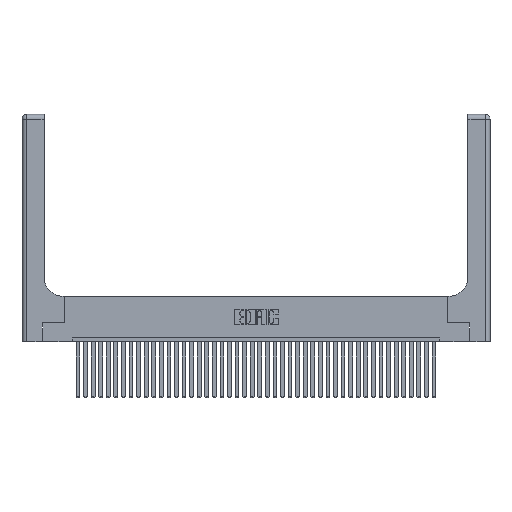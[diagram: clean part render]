
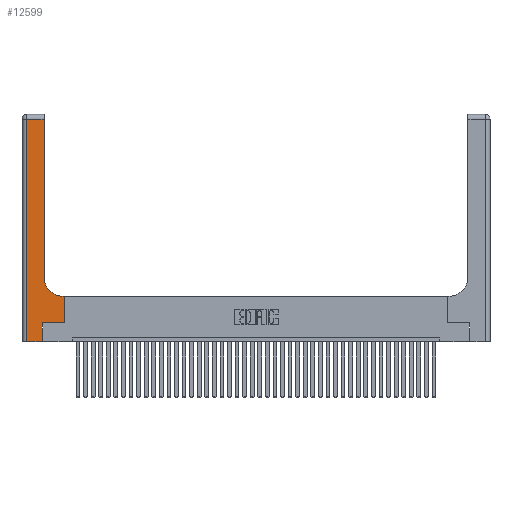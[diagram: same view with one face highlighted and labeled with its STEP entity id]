
A CAD part, top view. The second image highlights one B-rep face of the part: STEP entity #12599.
In plain terms, the highlighted planar face has unit normal (0, 0, 1).
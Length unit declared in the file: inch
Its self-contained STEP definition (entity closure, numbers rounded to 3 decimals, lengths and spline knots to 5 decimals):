
#260 = VERTEX_POINT ( 'NONE', #9766 ) ;
#655 = ORIENTED_EDGE ( 'NONE', *, *, #10106, .T. ) ;
#950 = VECTOR ( 'NONE', #1909, 39.37008 ) ;
#1289 = EDGE_CURVE ( 'NONE', #20110, #16293, #19134, .T. ) ;
#1830 = VECTOR ( 'NONE', #33829, 39.37008 ) ;
#1909 = DIRECTION ( 'NONE',  ( 0., 1., 0. ) ) ;
#2022 = LINE ( 'NONE', #32193, #34134 ) ;
#2368 = VERTEX_POINT ( 'NONE', #9151 ) ;
#2588 = EDGE_CURVE ( 'NONE', #7541, #29106, #37023, .T. ) ;
#3739 = AXIS2_PLACEMENT_3D ( 'NONE', #8335, #23676, #23802 ) ;
#3783 = DIRECTION ( 'NONE',  ( 0., 1., 0. ) ) ;
#4056 = CARTESIAN_POINT ( 'NONE',  ( 0.5585, 0.25, 0.37 ) ) ;
#4335 = CARTESIAN_POINT ( 'NONE',  ( 0.06, 0., 0.37 ) ) ;
#4371 = CARTESIAN_POINT ( 'NONE',  ( 0.5415, 0.6, 0.37 ) ) ;
#5521 = CARTESIAN_POINT ( 'NONE',  ( 0.2915, 3., 0.37 ) ) ;
#5650 = VERTEX_POINT ( 'NONE', #13972 ) ;
#7311 = ORIENTED_EDGE ( 'NONE', *, *, #1289, .T. ) ;
#7541 = VERTEX_POINT ( 'NONE', #4335 ) ;
#7920 = LINE ( 'NONE', #4056, #24430 ) ;
#7970 = PLANE ( 'NONE',  #15877 ) ;
#8243 = DIRECTION ( 'NONE',  ( -1., 0., 0. ) ) ;
#8335 = CARTESIAN_POINT ( 'NONE',  ( 0.5415, 0.85, 0.37 ) ) ;
#8697 = CARTESIAN_POINT ( 'NONE',  ( 0.06, 2.94, 0.37 ) ) ;
#8712 = EDGE_CURVE ( 'NONE', #29106, #5650, #25763, .T. ) ;
#8797 = DIRECTION ( 'NONE',  ( 0., 1., 0. ) ) ;
#8960 = VECTOR ( 'NONE', #8243, 39.37008 ) ;
#9113 = VERTEX_POINT ( 'NONE', #38278 ) ;
#9151 = CARTESIAN_POINT ( 'NONE',  ( 0.5585, 0.6, 0.37 ) ) ;
#9394 = VERTEX_POINT ( 'NONE', #4371 ) ;
#9766 = CARTESIAN_POINT ( 'NONE',  ( 0.5585, 0.25, 0.37 ) ) ;
#10106 = EDGE_CURVE ( 'NONE', #5650, #260, #18823, .T. ) ;
#10140 = LINE ( 'NONE', #15450, #1830 ) ;
#11658 = LINE ( 'NONE', #5521, #38415 ) ;
#12041 = VECTOR ( 'NONE', #24176, 39.37008 ) ;
#12599 = ADVANCED_FACE ( 'NONE', ( #38311 ), #7970, .F. ) ;
#13257 = EDGE_LOOP ( 'NONE', ( #27137, #7311, #25220, #32534, #21971, #655, #25902, #14515, #19451 ) ) ;
#13972 = CARTESIAN_POINT ( 'NONE',  ( 0.269, 0.25, 0.37 ) ) ;
#14515 = ORIENTED_EDGE ( 'NONE', *, *, #31595, .T. ) ;
#14566 = CIRCLE ( 'NONE', #3739, 0.25 ) ;
#15344 = EDGE_CURVE ( 'NONE', #16293, #7541, #2022, .T. ) ;
#15450 = CARTESIAN_POINT ( 'NONE',  ( 0.2915, 0.6, 0.37 ) ) ;
#15877 = AXIS2_PLACEMENT_3D ( 'NONE', #26570, #30076, #17301 ) ;
#16293 = VERTEX_POINT ( 'NONE', #8697 ) ;
#16333 = EDGE_CURVE ( 'NONE', #9394, #9113, #14566, .T. ) ;
#17215 = CARTESIAN_POINT ( 'NONE',  ( 0.269, 0., 0.37 ) ) ;
#17301 = DIRECTION ( 'NONE',  ( -1., 0., 0. ) ) ;
#18183 = CARTESIAN_POINT ( 'NONE',  ( 0.269, 0.25, 0.37 ) ) ;
#18823 = LINE ( 'NONE', #18183, #12041 ) ;
#18852 = EDGE_CURVE ( 'NONE', #260, #2368, #7920, .T. ) ;
#19134 = LINE ( 'NONE', #23717, #8960 ) ;
#19451 = ORIENTED_EDGE ( 'NONE', *, *, #16333, .T. ) ;
#20110 = VERTEX_POINT ( 'NONE', #30692 ) ;
#20945 = DIRECTION ( 'NONE',  ( 1., 0., 0. ) ) ;
#21940 = VECTOR ( 'NONE', #20945, 39.37008 ) ;
#21971 = ORIENTED_EDGE ( 'NONE', *, *, #8712, .T. ) ;
#23401 = CARTESIAN_POINT ( 'NONE',  ( 0.269, 0., 0.37 ) ) ;
#23676 = DIRECTION ( 'NONE',  ( 0., 0., -1. ) ) ;
#23717 = CARTESIAN_POINT ( 'NONE',  ( 0., 2.94, 0.37 ) ) ;
#23802 = DIRECTION ( 'NONE',  ( 1., 0., 0. ) ) ;
#24176 = DIRECTION ( 'NONE',  ( 1., 0., 0. ) ) ;
#24430 = VECTOR ( 'NONE', #3783, 39.37008 ) ;
#25220 = ORIENTED_EDGE ( 'NONE', *, *, #15344, .T. ) ;
#25683 = DIRECTION ( 'NONE',  ( 0., -1., 0. ) ) ;
#25763 = LINE ( 'NONE', #23401, #950 ) ;
#25902 = ORIENTED_EDGE ( 'NONE', *, *, #18852, .T. ) ;
#26570 = CARTESIAN_POINT ( 'NONE',  ( 0., 3., 0.37 ) ) ;
#27137 = ORIENTED_EDGE ( 'NONE', *, *, #39859, .T. ) ;
#29106 = VERTEX_POINT ( 'NONE', #17215 ) ;
#30076 = DIRECTION ( 'NONE',  ( 0., 0., -1. ) ) ;
#30692 = CARTESIAN_POINT ( 'NONE',  ( 0.2915, 2.94, 0.37 ) ) ;
#31595 = EDGE_CURVE ( 'NONE', #2368, #9394, #10140, .T. ) ;
#32193 = CARTESIAN_POINT ( 'NONE',  ( 0.06, 3., 0.37 ) ) ;
#32534 = ORIENTED_EDGE ( 'NONE', *, *, #2588, .T. ) ;
#33829 = DIRECTION ( 'NONE',  ( -1., 0., 0. ) ) ;
#34134 = VECTOR ( 'NONE', #25683, 39.37008 ) ;
#36481 = CARTESIAN_POINT ( 'NONE',  ( 0., 0., 0.37 ) ) ;
#37023 = LINE ( 'NONE', #36481, #21940 ) ;
#38278 = CARTESIAN_POINT ( 'NONE',  ( 0.2915, 0.85, 0.37 ) ) ;
#38311 = FACE_OUTER_BOUND ( 'NONE', #13257, .T. ) ;
#38415 = VECTOR ( 'NONE', #8797, 39.37008 ) ;
#39859 = EDGE_CURVE ( 'NONE', #9113, #20110, #11658, .T. ) ;
